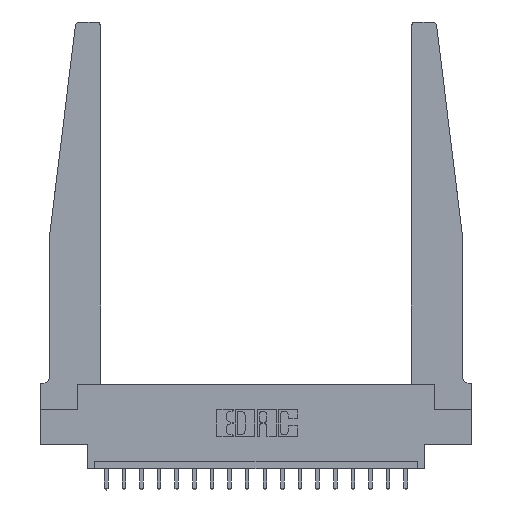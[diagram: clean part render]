
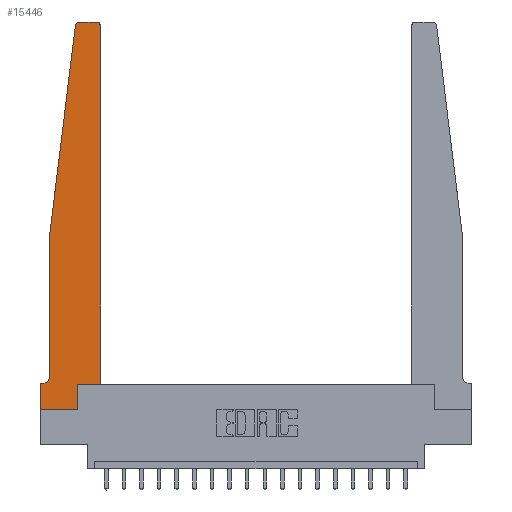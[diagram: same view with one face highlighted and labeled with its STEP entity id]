
A CAD part, top view. The second image highlights one B-rep face of the part: STEP entity #15446.
In plain terms, the highlighted planar face has unit normal (0, 0, 1).
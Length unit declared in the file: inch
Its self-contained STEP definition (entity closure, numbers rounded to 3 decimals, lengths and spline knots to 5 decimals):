
#9 = VECTOR ( 'NONE', #11483, 39.37008 ) ;
#1117 = CARTESIAN_POINT ( 'NONE',  ( 0.425, 0.18, 0.37 ) ) ;
#1287 = EDGE_CURVE ( 'NONE', #10411, #10118, #15405, .T. ) ;
#1502 = CARTESIAN_POINT ( 'NONE',  ( 0., 0., 0.37 ) ) ;
#1618 = LINE ( 'NONE', #11450, #8616 ) ;
#1697 = EDGE_CURVE ( 'NONE', #10642, #10645, #9365, .T. ) ;
#2018 = VERTEX_POINT ( 'NONE', #1117 ) ;
#2168 = ORIENTED_EDGE ( 'NONE', *, *, #3564, .T. ) ;
#2252 = EDGE_CURVE ( 'NONE', #5287, #10411, #6959, .T. ) ;
#2393 = CARTESIAN_POINT ( 'NONE',  ( 0.2605, 0.18, 0.37 ) ) ;
#2492 = AXIS2_PLACEMENT_3D ( 'NONE', #17763, #19272, #16345 ) ;
#2605 = CIRCLE ( 'NONE', #4711, 0.05 ) ;
#2784 = CARTESIAN_POINT ( 'NONE',  ( 0.065, 0.1875, 0.37 ) ) ;
#2906 = DIRECTION ( 'NONE',  ( -1., 0., 0. ) ) ;
#2953 = DIRECTION ( 'NONE',  ( 0., -1., 0. ) ) ;
#3308 = ORIENTED_EDGE ( 'NONE', *, *, #16216, .T. ) ;
#3564 = EDGE_CURVE ( 'NONE', #13924, #10642, #18843, .T. ) ;
#4194 = VECTOR ( 'NONE', #6815, 39.37008 ) ;
#4402 = VECTOR ( 'NONE', #4457, 39.37008 ) ;
#4457 = DIRECTION ( 'NONE',  ( 1., 0., 0. ) ) ;
#4478 = CARTESIAN_POINT ( 'NONE',  ( 0.24675, 2.72367, 0.37 ) ) ;
#4494 = ORIENTED_EDGE ( 'NONE', *, *, #11632, .T. ) ;
#4522 = LINE ( 'NONE', #9517, #15967 ) ;
#4651 = ORIENTED_EDGE ( 'NONE', *, *, #15135, .T. ) ;
#4687 = EDGE_CURVE ( 'NONE', #15979, #12723, #12740, .T. ) ;
#4711 = AXIS2_PLACEMENT_3D ( 'NONE', #15406, #12672, #15468 ) ;
#4800 = CARTESIAN_POINT ( 'NONE',  ( 0.065, 0.2375, 0.37 ) ) ;
#4895 = ORIENTED_EDGE ( 'NONE', *, *, #17632, .T. ) ;
#5287 = VERTEX_POINT ( 'NONE', #13294 ) ;
#5497 = VERTEX_POINT ( 'NONE', #8589 ) ;
#6181 = CIRCLE ( 'NONE', #6391, 0.03 ) ;
#6345 = CARTESIAN_POINT ( 'NONE',  ( 0.395, 2.75, 0.37 ) ) ;
#6391 = AXIS2_PLACEMENT_3D ( 'NONE', #8823, #11808, #19288 ) ;
#6683 = DIRECTION ( 'NONE',  ( 0., 0., 1. ) ) ;
#6815 = DIRECTION ( 'NONE',  ( 1., 0., 0. ) ) ;
#6816 = DIRECTION ( 'NONE',  ( -1., 0., 0. ) ) ;
#6959 = LINE ( 'NONE', #11926, #4402 ) ;
#6961 = CARTESIAN_POINT ( 'NONE',  ( 0.065, 1.25, 0.37 ) ) ;
#7195 = ORIENTED_EDGE ( 'NONE', *, *, #2252, .T. ) ;
#7229 = ORIENTED_EDGE ( 'NONE', *, *, #7359, .T. ) ;
#7359 = EDGE_CURVE ( 'NONE', #5497, #5287, #11889, .T. ) ;
#7732 = VECTOR ( 'NONE', #17129, 39.37008 ) ;
#7864 = ORIENTED_EDGE ( 'NONE', *, *, #1287, .T. ) ;
#7974 = VERTEX_POINT ( 'NONE', #18331 ) ;
#8065 = FACE_OUTER_BOUND ( 'NONE', #9494, .T. ) ;
#8403 = CARTESIAN_POINT ( 'NONE',  ( 0.065, 1.25, 0.37 ) ) ;
#8589 = CARTESIAN_POINT ( 'NONE',  ( 0., 0.1875, 0.37 ) ) ;
#8616 = VECTOR ( 'NONE', #6816, 39.37008 ) ;
#8736 = CARTESIAN_POINT ( 'NONE',  ( 0.2605, 0., 0.37 ) ) ;
#8823 = CARTESIAN_POINT ( 'NONE',  ( 0.27653, 2.72, 0.37 ) ) ;
#8876 = PLANE ( 'NONE',  #2492 ) ;
#9090 = VECTOR ( 'NONE', #2953, 39.37008 ) ;
#9182 = AXIS2_PLACEMENT_3D ( 'NONE', #12564, #6683, #11263 ) ;
#9365 = LINE ( 'NONE', #17064, #7732 ) ;
#9420 = VECTOR ( 'NONE', #2906, 39.37008 ) ;
#9494 = EDGE_LOOP ( 'NONE', ( #10863, #4651, #2168, #14339, #4494, #4895, #7229, #7195, #7864, #17218, #3308, #13651 ) ) ;
#9517 = CARTESIAN_POINT ( 'NONE',  ( 0.425, 0.18, 0.37 ) ) ;
#10118 = VERTEX_POINT ( 'NONE', #2393 ) ;
#10411 = VERTEX_POINT ( 'NONE', #8736 ) ;
#10642 = VERTEX_POINT ( 'NONE', #6961 ) ;
#10645 = VERTEX_POINT ( 'NONE', #4800 ) ;
#10863 = ORIENTED_EDGE ( 'NONE', *, *, #13260, .T. ) ;
#11263 = DIRECTION ( 'NONE',  ( 1., 0., 0. ) ) ;
#11266 = CARTESIAN_POINT ( 'NONE',  ( 0.425, 0.18, 0.37 ) ) ;
#11426 = VERTEX_POINT ( 'NONE', #18884 ) ;
#11450 = CARTESIAN_POINT ( 'NONE',  ( 0.25, 2.75, 0.37 ) ) ;
#11483 = DIRECTION ( 'NONE',  ( 0., 1., 0. ) ) ;
#11632 = EDGE_CURVE ( 'NONE', #10645, #7974, #2605, .T. ) ;
#11808 = DIRECTION ( 'NONE',  ( 0., 0., 1. ) ) ;
#11889 = LINE ( 'NONE', #1502, #9090 ) ;
#11926 = CARTESIAN_POINT ( 'NONE',  ( 0., 0., 0.37 ) ) ;
#12106 = VECTOR ( 'NONE', #12898, 39.37008 ) ;
#12175 = LINE ( 'NONE', #11266, #4194 ) ;
#12564 = CARTESIAN_POINT ( 'NONE',  ( 0.395, 2.72, 0.37 ) ) ;
#12672 = DIRECTION ( 'NONE',  ( 0., 0., -1. ) ) ;
#12723 = VERTEX_POINT ( 'NONE', #6345 ) ;
#12740 = CIRCLE ( 'NONE', #9182, 0.03 ) ;
#12898 = DIRECTION ( 'NONE',  ( -0.122, -0.992, 0. ) ) ;
#13260 = EDGE_CURVE ( 'NONE', #12723, #11426, #1618, .T. ) ;
#13294 = CARTESIAN_POINT ( 'NONE',  ( 0., 0., 0.37 ) ) ;
#13651 = ORIENTED_EDGE ( 'NONE', *, *, #4687, .T. ) ;
#13924 = VERTEX_POINT ( 'NONE', #4478 ) ;
#13968 = DIRECTION ( 'NONE',  ( 0., 1., 0. ) ) ;
#14339 = ORIENTED_EDGE ( 'NONE', *, *, #1697, .T. ) ;
#14985 = LINE ( 'NONE', #2784, #9420 ) ;
#15135 = EDGE_CURVE ( 'NONE', #11426, #13924, #6181, .T. ) ;
#15405 = LINE ( 'NONE', #17405, #9 ) ;
#15406 = CARTESIAN_POINT ( 'NONE',  ( 0.015, 0.2375, 0.37 ) ) ;
#15446 = ADVANCED_FACE ( 'NONE', ( #8065 ), #8876, .T. ) ;
#15468 = DIRECTION ( 'NONE',  ( -1., 0., 0. ) ) ;
#15967 = VECTOR ( 'NONE', #13968, 39.37008 ) ;
#15979 = VERTEX_POINT ( 'NONE', #18482 ) ;
#16216 = EDGE_CURVE ( 'NONE', #2018, #15979, #4522, .T. ) ;
#16345 = DIRECTION ( 'NONE',  ( 1., 0., 0. ) ) ;
#17064 = CARTESIAN_POINT ( 'NONE',  ( 0.065, 1.25, 0.37 ) ) ;
#17129 = DIRECTION ( 'NONE',  ( 0., -1., 0. ) ) ;
#17218 = ORIENTED_EDGE ( 'NONE', *, *, #18579, .T. ) ;
#17405 = CARTESIAN_POINT ( 'NONE',  ( 0.2605, 0.18, 0.37 ) ) ;
#17632 = EDGE_CURVE ( 'NONE', #7974, #5497, #14985, .T. ) ;
#17763 = CARTESIAN_POINT ( 'NONE',  ( 0., 0.1875, 0.37 ) ) ;
#18331 = CARTESIAN_POINT ( 'NONE',  ( 0.015, 0.1875, 0.37 ) ) ;
#18482 = CARTESIAN_POINT ( 'NONE',  ( 0.425, 2.72, 0.37 ) ) ;
#18579 = EDGE_CURVE ( 'NONE', #10118, #2018, #12175, .T. ) ;
#18843 = LINE ( 'NONE', #8403, #12106 ) ;
#18884 = CARTESIAN_POINT ( 'NONE',  ( 0.27653, 2.75, 0.37 ) ) ;
#19272 = DIRECTION ( 'NONE',  ( 0., 0., 1. ) ) ;
#19288 = DIRECTION ( 'NONE',  ( 1., 0., 0. ) ) ;
